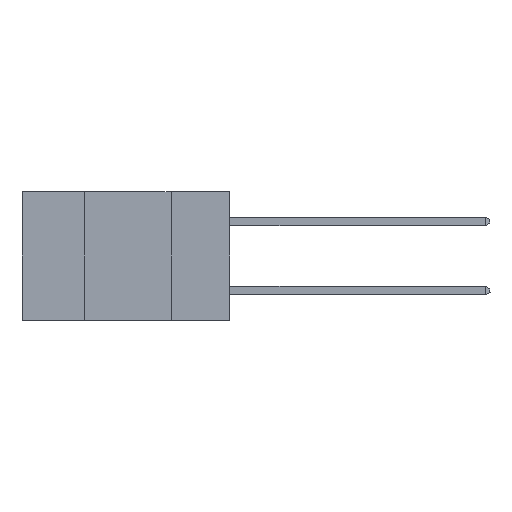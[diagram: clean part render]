
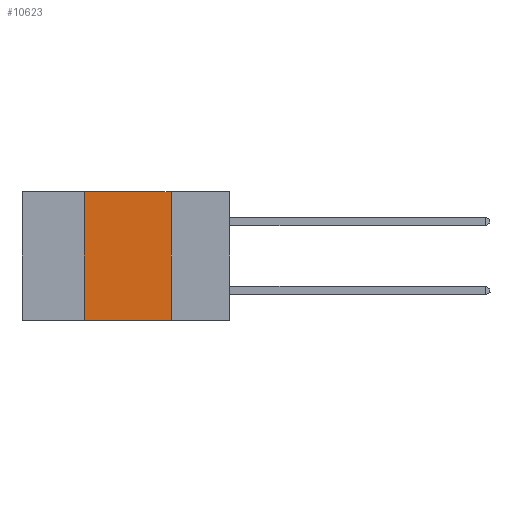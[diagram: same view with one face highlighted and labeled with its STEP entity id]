
A CAD part, left-side view. The second image highlights one B-rep face of the part: STEP entity #10623.
In plain terms, the highlighted planar face has unit normal (-1, 0, 0).
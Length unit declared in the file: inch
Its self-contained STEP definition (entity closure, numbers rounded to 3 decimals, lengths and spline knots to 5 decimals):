
#309 = VERTEX_POINT ( 'NONE', #14818 ) ;
#340 = AXIS2_PLACEMENT_3D ( 'NONE', #4298, #26772, #21826 ) ;
#533 = VERTEX_POINT ( 'NONE', #23608 ) ;
#1099 = EDGE_LOOP ( 'NONE', ( #13452, #20201, #23181, #8922 ) ) ;
#1724 = DIRECTION ( 'NONE',  ( 0., -1., 0. ) ) ;
#2563 = LINE ( 'NONE', #6194, #19804 ) ;
#4298 = CARTESIAN_POINT ( 'NONE',  ( 0., 0.6, 0. ) ) ;
#4406 = VERTEX_POINT ( 'NONE', #26553 ) ;
#4719 = VECTOR ( 'NONE', #23601, 39.37008 ) ;
#6074 = CARTESIAN_POINT ( 'NONE',  ( 0., 0.42, 0. ) ) ;
#6194 = CARTESIAN_POINT ( 'NONE',  ( 0., 0.6, 0. ) ) ;
#6225 = VERTEX_POINT ( 'NONE', #17415 ) ;
#8922 = ORIENTED_EDGE ( 'NONE', *, *, #10065, .T. ) ;
#9802 = LINE ( 'NONE', #6074, #4719 ) ;
#10065 = EDGE_CURVE ( 'NONE', #4406, #309, #30985, .T. ) ;
#10623 = ADVANCED_FACE ( 'NONE', ( #28242 ), #16694, .F. ) ;
#13452 = ORIENTED_EDGE ( 'NONE', *, *, #28387, .F. ) ;
#13699 = CARTESIAN_POINT ( 'NONE',  ( 0., 0.17, 0. ) ) ;
#14818 = CARTESIAN_POINT ( 'NONE',  ( 0., 0.17, -0.37 ) ) ;
#16694 = PLANE ( 'NONE',  #340 ) ;
#16882 = VECTOR ( 'NONE', #18611, 39.37008 ) ;
#17415 = CARTESIAN_POINT ( 'NONE',  ( 0., 0.17, 0. ) ) ;
#18611 = DIRECTION ( 'NONE',  ( 0., 0., -1. ) ) ;
#19804 = VECTOR ( 'NONE', #1724, 39.37008 ) ;
#20201 = ORIENTED_EDGE ( 'NONE', *, *, #24948, .F. ) ;
#21826 = DIRECTION ( 'NONE',  ( 0., 0., -1. ) ) ;
#23181 = ORIENTED_EDGE ( 'NONE', *, *, #28658, .F. ) ;
#23601 = DIRECTION ( 'NONE',  ( 0., 0., 1. ) ) ;
#23608 = CARTESIAN_POINT ( 'NONE',  ( 0., 0.42, 0. ) ) ;
#24302 = VECTOR ( 'NONE', #25742, 39.37008 ) ;
#24948 = EDGE_CURVE ( 'NONE', #533, #6225, #2563, .T. ) ;
#25742 = DIRECTION ( 'NONE',  ( 0., -1., 0. ) ) ;
#26553 = CARTESIAN_POINT ( 'NONE',  ( 0., 0.42, -0.37 ) ) ;
#26772 = DIRECTION ( 'NONE',  ( 1., 0., 0. ) ) ;
#27863 = LINE ( 'NONE', #13699, #16882 ) ;
#28242 = FACE_OUTER_BOUND ( 'NONE', #1099, .T. ) ;
#28387 = EDGE_CURVE ( 'NONE', #6225, #309, #27863, .T. ) ;
#28658 = EDGE_CURVE ( 'NONE', #4406, #533, #9802, .T. ) ;
#30985 = LINE ( 'NONE', #31113, #24302 ) ;
#31113 = CARTESIAN_POINT ( 'NONE',  ( 0., 0.6, -0.37 ) ) ;
